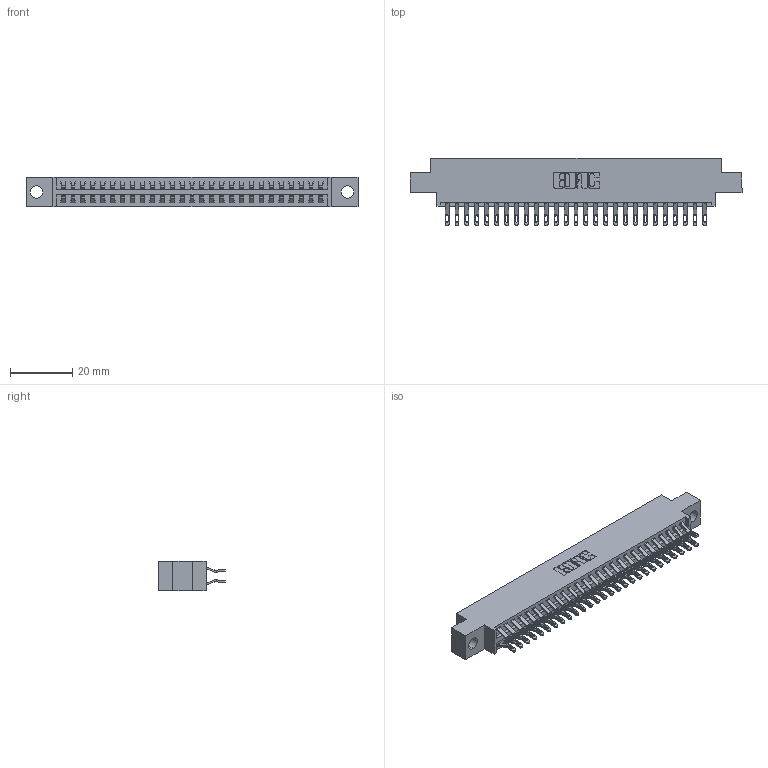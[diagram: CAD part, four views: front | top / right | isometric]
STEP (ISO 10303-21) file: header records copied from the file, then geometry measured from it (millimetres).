
FILE_DESCRIPTION (( 'STEP AP203' ), '1' );
FILE_NAME ('346-054-555-804.STEP', '2022-05-21T03:53:40', ( '' ), ( '' ), 'SwSTEP 2.0', 'SolidWorks 2020', '' );
FILE_SCHEMA (( 'CONFIG_CONTROL_DESIGN' ));
Length unit declared in the file: inch
Products named in the file (3): 345-292-001_555 Tail; 346 Part_0.170 Offset - 0.156 Dia-TH; 346-054-555-804
Assembly tree (55 placements, depth 2):
  346-054-555-804
    346 Part_0.170 Offset - 0.156 Dia-TH
    345-292-001_555 Tail  x54
Bounding box: 106.3 x 21.46 x 9.4 mm (x, y, z)
Volume: 10145 mm3; surface area: 14295.1 mm2
Topology: 55 solids, 55 shells, 3272 faces, 10259 edges, 6838 vertices
Faces by surface type: plane 1876, cylinder 1396
Entity records: 20517 total; most frequent: CARTESIAN_POINT 3444, ORIENTED_EDGE 3346, DIRECTION 3053, EDGE_CURVE 1673, LINE 1413, VECTOR 1413, VERTEX_POINT 1114, AXIS2_PLACEMENT_3D 820
